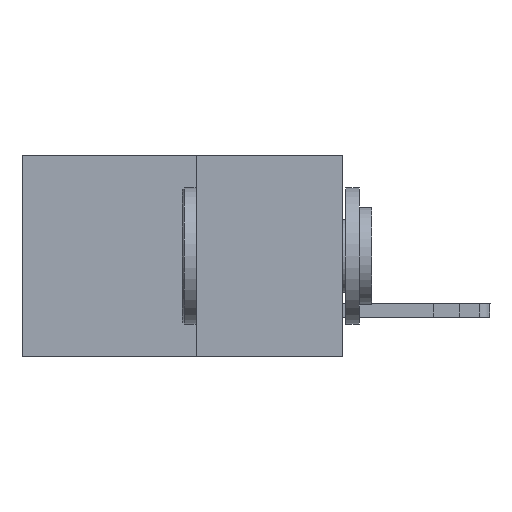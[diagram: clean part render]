
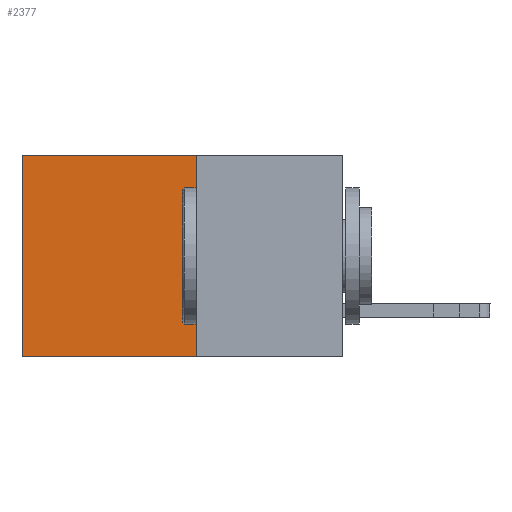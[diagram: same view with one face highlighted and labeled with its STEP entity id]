
A CAD part, left-side view. The second image highlights one B-rep face of the part: STEP entity #2377.
In plain terms, the highlighted planar face has unit normal (-1, 0, 0).
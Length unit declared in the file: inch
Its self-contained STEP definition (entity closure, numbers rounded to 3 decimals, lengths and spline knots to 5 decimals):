
#315 = DIRECTION ( 'NONE',  ( 0., 0., -1. ) ) ;
#791 = VERTEX_POINT ( 'NONE', #17661 ) ;
#1736 = EDGE_CURVE ( 'NONE', #8725, #12818, #12538, .T. ) ;
#2377 = ADVANCED_FACE ( 'NONE', ( #14398 ), #11156, .F. ) ;
#4200 = AXIS2_PLACEMENT_3D ( 'NONE', #11159, #10832, #10744 ) ;
#4533 = LINE ( 'NONE', #4771, #15787 ) ;
#4771 = CARTESIAN_POINT ( 'NONE',  ( 0.277, 0.27, -0.37 ) ) ;
#4906 = VECTOR ( 'NONE', #12501, 39.37008 ) ;
#5298 = VERTEX_POINT ( 'NONE', #11394 ) ;
#6276 = CARTESIAN_POINT ( 'NONE',  ( 0.277, 0.59, 0. ) ) ;
#7023 = VECTOR ( 'NONE', #11368, 39.37008 ) ;
#7750 = EDGE_LOOP ( 'NONE', ( #8913, #12008, #9159, #17090 ) ) ;
#8234 = EDGE_CURVE ( 'NONE', #8725, #5298, #14477, .T. ) ;
#8725 = VERTEX_POINT ( 'NONE', #14279 ) ;
#8913 = ORIENTED_EDGE ( 'NONE', *, *, #11231, .T. ) ;
#9137 = DIRECTION ( 'NONE',  ( 0., 1., 0. ) ) ;
#9159 = ORIENTED_EDGE ( 'NONE', *, *, #8234, .F. ) ;
#10744 = DIRECTION ( 'NONE',  ( 0., 0., -1. ) ) ;
#10832 = DIRECTION ( 'NONE',  ( 1., 0., 0. ) ) ;
#11156 = PLANE ( 'NONE',  #4200 ) ;
#11159 = CARTESIAN_POINT ( 'NONE',  ( 0.277, 0.27, -0.37 ) ) ;
#11231 = EDGE_CURVE ( 'NONE', #12818, #791, #14449, .T. ) ;
#11368 = DIRECTION ( 'NONE',  ( 0., 0., -1. ) ) ;
#11394 = CARTESIAN_POINT ( 'NONE',  ( 0.277, 0.27, -0.37 ) ) ;
#12008 = ORIENTED_EDGE ( 'NONE', *, *, #15943, .F. ) ;
#12501 = DIRECTION ( 'NONE',  ( 0., 1., 0. ) ) ;
#12538 = LINE ( 'NONE', #17888, #4906 ) ;
#12818 = VERTEX_POINT ( 'NONE', #6276 ) ;
#13641 = VECTOR ( 'NONE', #315, 39.37008 ) ;
#14279 = CARTESIAN_POINT ( 'NONE',  ( 0.277, 0.27, 0. ) ) ;
#14398 = FACE_OUTER_BOUND ( 'NONE', #7750, .T. ) ;
#14449 = LINE ( 'NONE', #15381, #7023 ) ;
#14477 = LINE ( 'NONE', #14654, #13641 ) ;
#14654 = CARTESIAN_POINT ( 'NONE',  ( 0.277, 0.27, -0.37 ) ) ;
#15381 = CARTESIAN_POINT ( 'NONE',  ( 0.277, 0.59, -0.37 ) ) ;
#15787 = VECTOR ( 'NONE', #9137, 39.37008 ) ;
#15943 = EDGE_CURVE ( 'NONE', #5298, #791, #4533, .T. ) ;
#17090 = ORIENTED_EDGE ( 'NONE', *, *, #1736, .T. ) ;
#17661 = CARTESIAN_POINT ( 'NONE',  ( 0.277, 0.59, -0.37 ) ) ;
#17888 = CARTESIAN_POINT ( 'NONE',  ( 0.277, 0.27, 0. ) ) ;
